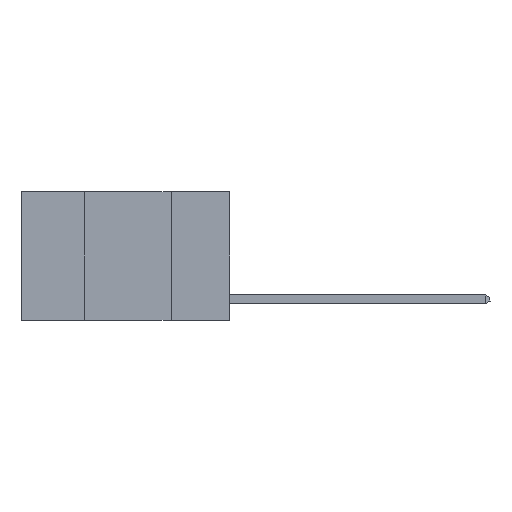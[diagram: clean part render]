
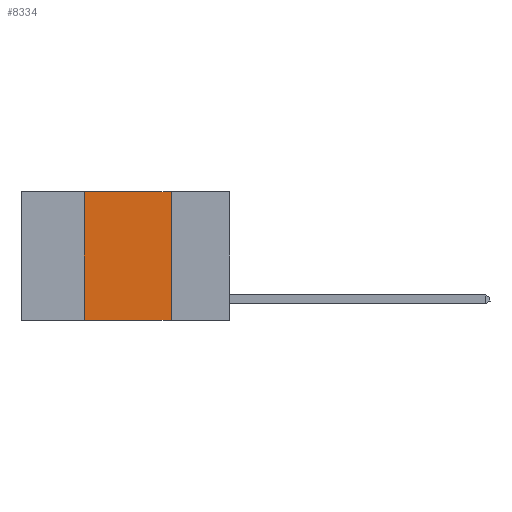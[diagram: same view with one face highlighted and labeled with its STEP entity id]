
A CAD part, left-side view. The second image highlights one B-rep face of the part: STEP entity #8334.
In plain terms, the highlighted planar face has unit normal (-1, 0, 0).
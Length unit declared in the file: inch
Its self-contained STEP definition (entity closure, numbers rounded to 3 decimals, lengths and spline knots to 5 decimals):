
#120 = CARTESIAN_POINT ( 'NONE',  ( 0., 0.42, -0.37 ) ) ;
#480 = DIRECTION ( 'NONE',  ( 0., -1., 0. ) ) ;
#801 = VECTOR ( 'NONE', #2672, 39.37008 ) ;
#2233 = EDGE_CURVE ( 'NONE', #14870, #15546, #4578, .T. ) ;
#2389 = FACE_OUTER_BOUND ( 'NONE', #11701, .T. ) ;
#2672 = DIRECTION ( 'NONE',  ( 0., 0., -1. ) ) ;
#4155 = EDGE_CURVE ( 'NONE', #12003, #14870, #9536, .T. ) ;
#4383 = DIRECTION ( 'NONE',  ( 0., -1., 0. ) ) ;
#4578 = LINE ( 'NONE', #6654, #801 ) ;
#4584 = CARTESIAN_POINT ( 'NONE',  ( 0., 0.42, 0. ) ) ;
#4769 = VECTOR ( 'NONE', #16116, 39.37008 ) ;
#4827 = LINE ( 'NONE', #5491, #11680 ) ;
#5491 = CARTESIAN_POINT ( 'NONE',  ( 0., 0.6, -0.37 ) ) ;
#5849 = ORIENTED_EDGE ( 'NONE', *, *, #7158, .T. ) ;
#6525 = VERTEX_POINT ( 'NONE', #120 ) ;
#6654 = CARTESIAN_POINT ( 'NONE',  ( 0., 0.17, 0. ) ) ;
#7158 = EDGE_CURVE ( 'NONE', #6525, #15546, #4827, .T. ) ;
#7314 = VECTOR ( 'NONE', #4383, 39.37008 ) ;
#7875 = ORIENTED_EDGE ( 'NONE', *, *, #14096, .F. ) ;
#8191 = LINE ( 'NONE', #4584, #4769 ) ;
#8334 = ADVANCED_FACE ( 'NONE', ( #2389 ), #11421, .F. ) ;
#9536 = LINE ( 'NONE', #15817, #7314 ) ;
#9578 = CARTESIAN_POINT ( 'NONE',  ( 0., 0.42, 0. ) ) ;
#9988 = AXIS2_PLACEMENT_3D ( 'NONE', #15474, #11367, #15363 ) ;
#10910 = ORIENTED_EDGE ( 'NONE', *, *, #2233, .F. ) ;
#11367 = DIRECTION ( 'NONE',  ( 1., 0., 0. ) ) ;
#11421 = PLANE ( 'NONE',  #9988 ) ;
#11680 = VECTOR ( 'NONE', #480, 39.37008 ) ;
#11701 = EDGE_LOOP ( 'NONE', ( #10910, #16015, #7875, #5849 ) ) ;
#12003 = VERTEX_POINT ( 'NONE', #9578 ) ;
#13859 = CARTESIAN_POINT ( 'NONE',  ( 0., 0.17, 0. ) ) ;
#14096 = EDGE_CURVE ( 'NONE', #6525, #12003, #8191, .T. ) ;
#14870 = VERTEX_POINT ( 'NONE', #13859 ) ;
#15363 = DIRECTION ( 'NONE',  ( 0., 0., -1. ) ) ;
#15474 = CARTESIAN_POINT ( 'NONE',  ( 0., 0.6, 0. ) ) ;
#15546 = VERTEX_POINT ( 'NONE', #16165 ) ;
#15817 = CARTESIAN_POINT ( 'NONE',  ( 0., 0.6, 0. ) ) ;
#16015 = ORIENTED_EDGE ( 'NONE', *, *, #4155, .F. ) ;
#16116 = DIRECTION ( 'NONE',  ( 0., 0., 1. ) ) ;
#16165 = CARTESIAN_POINT ( 'NONE',  ( 0., 0.17, -0.37 ) ) ;
